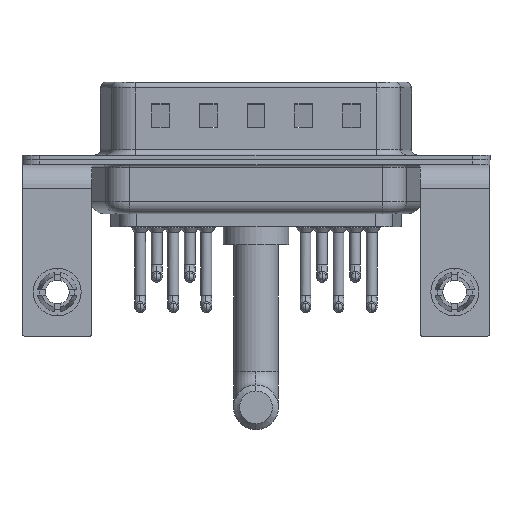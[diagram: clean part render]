
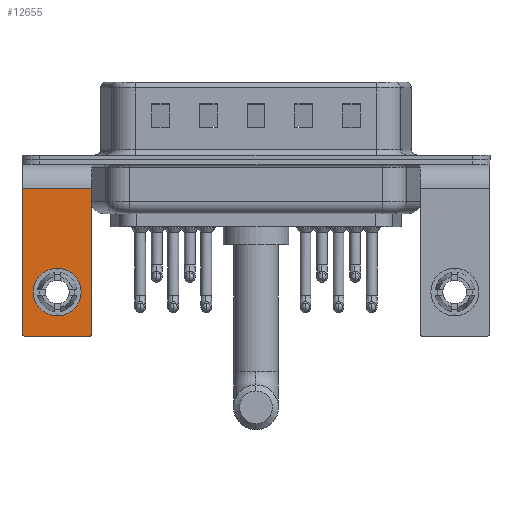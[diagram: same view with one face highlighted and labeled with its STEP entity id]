
A CAD part, front view. The second image highlights one B-rep face of the part: STEP entity #12655.
In plain terms, the highlighted planar face has unit normal (0, -1, 0).
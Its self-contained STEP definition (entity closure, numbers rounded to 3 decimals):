
#657 = CARTESIAN_POINT ( 'NONE',  ( -2.65, -6.25, -14.8 ) ) ;
#793 = DIRECTION ( 'NONE',  ( 0., -1., 0. ) ) ;
#871 = CIRCLE ( 'NONE', #1672, 0.25 ) ;
#1254 = VECTOR ( 'NONE', #2148, 1000. ) ;
#1326 = CARTESIAN_POINT ( 'NONE',  ( -2.9, -6.25, -14.55 ) ) ;
#1620 = FACE_OUTER_BOUND ( 'NONE', #16677, .T. ) ;
#1672 = AXIS2_PLACEMENT_3D ( 'NONE', #5560, #3946, #13832 ) ;
#1775 = EDGE_LOOP ( 'NONE', ( #13575, #10270 ) ) ;
#2024 = CARTESIAN_POINT ( 'NONE',  ( 2.65, -6.25, -14.8 ) ) ;
#2148 = DIRECTION ( 'NONE',  ( 0., 0., -1. ) ) ;
#2339 = ORIENTED_EDGE ( 'NONE', *, *, #8475, .T. ) ;
#2439 = ORIENTED_EDGE ( 'NONE', *, *, #5002, .T. ) ;
#2622 = CIRCLE ( 'NONE', #13813, 2. ) ;
#2892 = CARTESIAN_POINT ( 'NONE',  ( 0., -6.25, -9.07 ) ) ;
#3125 = AXIS2_PLACEMENT_3D ( 'NONE', #9255, #11508, #9369 ) ;
#3855 = DIRECTION ( 'NONE',  ( 0., 0., 1. ) ) ;
#3877 = EDGE_CURVE ( 'NONE', #18340, #7903, #16411, .T. ) ;
#3946 = DIRECTION ( 'NONE',  ( 0., -1., 0. ) ) ;
#4264 = EDGE_CURVE ( 'NONE', #20734, #16612, #20005, .T. ) ;
#4373 = LINE ( 'NONE', #23296, #1254 ) ;
#5002 = EDGE_CURVE ( 'NONE', #20734, #8626, #871, .T. ) ;
#5211 = ORIENTED_EDGE ( 'NONE', *, *, #15215, .F. ) ;
#5560 = CARTESIAN_POINT ( 'NONE',  ( 2.65, -6.25, -14.55 ) ) ;
#5707 = VECTOR ( 'NONE', #13270, 1000. ) ;
#5919 = EDGE_CURVE ( 'NONE', #7903, #18340, #2622, .T. ) ;
#6639 = CARTESIAN_POINT ( 'NONE',  ( 0., -6.25, -11.07 ) ) ;
#7307 = LINE ( 'NONE', #22464, #24759 ) ;
#7903 = VERTEX_POINT ( 'NONE', #2892 ) ;
#8475 = EDGE_CURVE ( 'NONE', #14235, #19775, #9267, .T. ) ;
#8626 = VERTEX_POINT ( 'NONE', #15520 ) ;
#8740 = CARTESIAN_POINT ( 'NONE',  ( 2.9, -6.25, -14.8 ) ) ;
#8892 = DIRECTION ( 'NONE',  ( 0., 1., 0. ) ) ;
#9228 = AXIS2_PLACEMENT_3D ( 'NONE', #6639, #8892, #18404 ) ;
#9255 = CARTESIAN_POINT ( 'NONE',  ( 2.9, -6.25, -2.4 ) ) ;
#9267 = LINE ( 'NONE', #14789, #5707 ) ;
#9369 = DIRECTION ( 'NONE',  ( 0., 0., 1. ) ) ;
#10270 = ORIENTED_EDGE ( 'NONE', *, *, #5919, .T. ) ;
#10494 = DIRECTION ( 'NONE',  ( -1., 0., 0. ) ) ;
#11508 = DIRECTION ( 'NONE',  ( 0., 1., 0. ) ) ;
#11783 = EDGE_CURVE ( 'NONE', #19775, #16612, #23906, .T. ) ;
#12179 = CARTESIAN_POINT ( 'NONE',  ( -2.65, -6.25, -14.55 ) ) ;
#12655 = ADVANCED_FACE ( 'NONE', ( #20870, #1620 ), #13132, .F. ) ;
#13132 = PLANE ( 'NONE',  #3125 ) ;
#13270 = DIRECTION ( 'NONE',  ( 0., 0., -1. ) ) ;
#13365 = CARTESIAN_POINT ( 'NONE',  ( 0., -6.25, -11.07 ) ) ;
#13487 = EDGE_CURVE ( 'NONE', #15943, #14235, #7307, .T. ) ;
#13575 = ORIENTED_EDGE ( 'NONE', *, *, #3877, .T. ) ;
#13813 = AXIS2_PLACEMENT_3D ( 'NONE', #13365, #20986, #3855 ) ;
#13832 = DIRECTION ( 'NONE',  ( 0., 0., 1. ) ) ;
#14171 = ORIENTED_EDGE ( 'NONE', *, *, #11783, .T. ) ;
#14235 = VERTEX_POINT ( 'NONE', #22377 ) ;
#14789 = CARTESIAN_POINT ( 'NONE',  ( -2.9, -6.25, -2.4 ) ) ;
#15215 = EDGE_CURVE ( 'NONE', #15943, #8626, #4373, .T. ) ;
#15520 = CARTESIAN_POINT ( 'NONE',  ( 2.9, -6.25, -14.55 ) ) ;
#15943 = VERTEX_POINT ( 'NONE', #20342 ) ;
#16023 = VECTOR ( 'NONE', #10494, 1000. ) ;
#16411 = CIRCLE ( 'NONE', #9228, 2. ) ;
#16610 = ORIENTED_EDGE ( 'NONE', *, *, #13487, .T. ) ;
#16612 = VERTEX_POINT ( 'NONE', #657 ) ;
#16677 = EDGE_LOOP ( 'NONE', ( #2339, #14171, #22286, #2439, #5211, #16610 ) ) ;
#18179 = DIRECTION ( 'NONE',  ( 0., 0., 1. ) ) ;
#18340 = VERTEX_POINT ( 'NONE', #18568 ) ;
#18404 = DIRECTION ( 'NONE',  ( 0., 0., 1. ) ) ;
#18561 = DIRECTION ( 'NONE',  ( -1., 0., 0. ) ) ;
#18568 = CARTESIAN_POINT ( 'NONE',  ( 0., -6.25, -13.07 ) ) ;
#19505 = AXIS2_PLACEMENT_3D ( 'NONE', #12179, #793, #18179 ) ;
#19775 = VERTEX_POINT ( 'NONE', #1326 ) ;
#20005 = LINE ( 'NONE', #8740, #16023 ) ;
#20342 = CARTESIAN_POINT ( 'NONE',  ( 2.9, -6.25, -2.4 ) ) ;
#20734 = VERTEX_POINT ( 'NONE', #2024 ) ;
#20870 = FACE_BOUND ( 'NONE', #1775, .T. ) ;
#20986 = DIRECTION ( 'NONE',  ( 0., 1., 0. ) ) ;
#22286 = ORIENTED_EDGE ( 'NONE', *, *, #4264, .F. ) ;
#22377 = CARTESIAN_POINT ( 'NONE',  ( -2.9, -6.25, -2.4 ) ) ;
#22464 = CARTESIAN_POINT ( 'NONE',  ( 2.9, -6.25, -2.4 ) ) ;
#23296 = CARTESIAN_POINT ( 'NONE',  ( 2.9, -6.25, -2.4 ) ) ;
#23906 = CIRCLE ( 'NONE', #19505, 0.25 ) ;
#24759 = VECTOR ( 'NONE', #18561, 1000. ) ;
